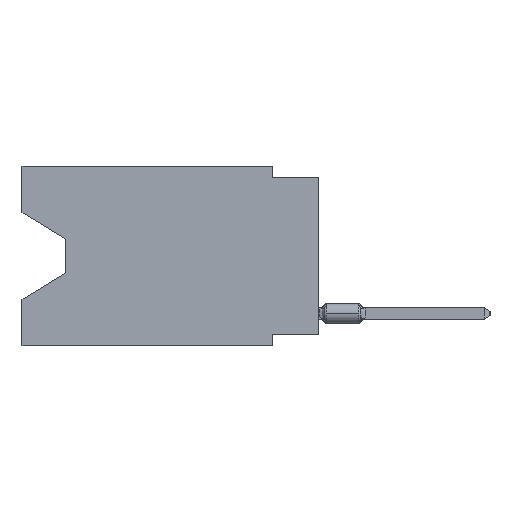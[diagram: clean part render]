
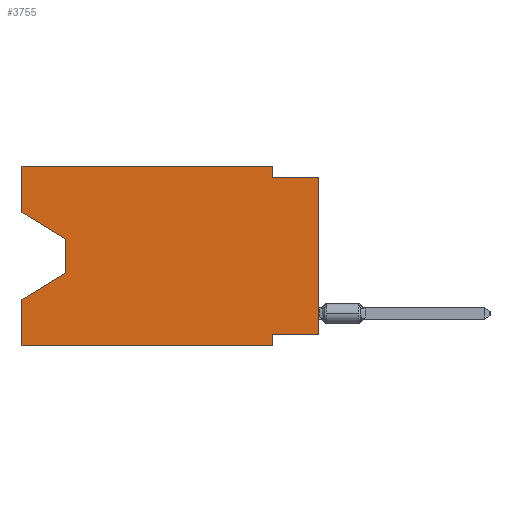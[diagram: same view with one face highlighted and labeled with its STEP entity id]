
A CAD part, left-side view. The second image highlights one B-rep face of the part: STEP entity #3755.
In plain terms, the highlighted planar face has unit normal (-1, 0, 0).
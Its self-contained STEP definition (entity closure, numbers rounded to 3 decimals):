
#475 = CARTESIAN_POINT ( 'NONE',  ( 0., 2.54, -9.906 ) ) ;
#576 = EDGE_CURVE ( 'NONE', #1018, #10502, #11870, .T. ) ;
#692 = ORIENTED_EDGE ( 'NONE', *, *, #12972, .T. ) ;
#781 = EDGE_CURVE ( 'NONE', #21900, #9035, #8437, .T. ) ;
#1018 = VERTEX_POINT ( 'NONE', #19758 ) ;
#1227 = DIRECTION ( 'NONE',  ( 1., 0., 0. ) ) ;
#1311 = LINE ( 'NONE', #3741, #22983 ) ;
#1366 = LINE ( 'NONE', #25809, #26081 ) ;
#2174 = ORIENTED_EDGE ( 'NONE', *, *, #20795, .F. ) ;
#2317 = VERTEX_POINT ( 'NONE', #19214 ) ;
#3523 = DIRECTION ( 'NONE',  ( 0., 0.855, -0.519 ) ) ;
#3629 = LINE ( 'NONE', #17887, #20017 ) ;
#3741 = CARTESIAN_POINT ( 'NONE',  ( 0., 16.383, -9.906 ) ) ;
#3755 = ADVANCED_FACE ( 'NONE', ( #15972 ), #15324, .F. ) ;
#3882 = VECTOR ( 'NONE', #12177, 1000. ) ;
#4515 = EDGE_CURVE ( 'NONE', #24877, #6491, #29339, .T. ) ;
#5330 = LINE ( 'NONE', #24775, #22508 ) ;
#5624 = CARTESIAN_POINT ( 'NONE',  ( 0., 13.97, -5.893 ) ) ;
#6162 = DIRECTION ( 'NONE',  ( 0., 0., -1. ) ) ;
#6491 = VERTEX_POINT ( 'NONE', #12184 ) ;
#6551 = VECTOR ( 'NONE', #9279, 1000. ) ;
#7434 = DIRECTION ( 'NONE',  ( 0., 0., -1. ) ) ;
#7887 = EDGE_CURVE ( 'NONE', #12983, #31976, #1311, .T. ) ;
#8037 = VECTOR ( 'NONE', #14557, 1000. ) ;
#8437 = LINE ( 'NONE', #10877, #13774 ) ;
#9035 = VERTEX_POINT ( 'NONE', #13782 ) ;
#9279 = DIRECTION ( 'NONE',  ( 0., 1., 0. ) ) ;
#9774 = EDGE_LOOP ( 'NONE', ( #692, #27074, #11202, #24869, #21378, #28714, #13624, #13614, #2174, #17462, #12701, #31090 ) ) ;
#9976 = VERTEX_POINT ( 'NONE', #17075 ) ;
#9989 = LINE ( 'NONE', #22144, #13260 ) ;
#10378 = VECTOR ( 'NONE', #13306, 1000. ) ;
#10423 = DIRECTION ( 'NONE',  ( 0., -0.855, -0.519 ) ) ;
#10435 = CARTESIAN_POINT ( 'NONE',  ( 0., 16.383, -2.546 ) ) ;
#10502 = VERTEX_POINT ( 'NONE', #13295 ) ;
#10621 = DIRECTION ( 'NONE',  ( 0., 0., -1. ) ) ;
#10664 = VECTOR ( 'NONE', #3523, 1000. ) ;
#10877 = CARTESIAN_POINT ( 'NONE',  ( 0., 13.97, -4.013 ) ) ;
#11202 = ORIENTED_EDGE ( 'NONE', *, *, #12556, .T. ) ;
#11345 = CARTESIAN_POINT ( 'NONE',  ( 0., 0., -0.635 ) ) ;
#11764 = EDGE_CURVE ( 'NONE', #10502, #31976, #20875, .T. ) ;
#11870 = LINE ( 'NONE', #19007, #6551 ) ;
#12008 = CARTESIAN_POINT ( 'NONE',  ( 0., 2.54, 0. ) ) ;
#12177 = DIRECTION ( 'NONE',  ( 0., 0., 1. ) ) ;
#12184 = CARTESIAN_POINT ( 'NONE',  ( 0., 16.383, 0. ) ) ;
#12424 = EDGE_CURVE ( 'NONE', #1018, #24943, #9989, .T. ) ;
#12425 = DIRECTION ( 'NONE',  ( 0., 0., 1. ) ) ;
#12556 = EDGE_CURVE ( 'NONE', #9035, #9976, #13536, .T. ) ;
#12701 = ORIENTED_EDGE ( 'NONE', *, *, #18022, .F. ) ;
#12972 = EDGE_CURVE ( 'NONE', #24877, #21900, #3629, .T. ) ;
#12983 = VERTEX_POINT ( 'NONE', #20468 ) ;
#13032 = CARTESIAN_POINT ( 'NONE',  ( 0., 0., -0.635 ) ) ;
#13260 = VECTOR ( 'NONE', #12425, 1000. ) ;
#13295 = CARTESIAN_POINT ( 'NONE',  ( 0., 2.54, -9.271 ) ) ;
#13306 = DIRECTION ( 'NONE',  ( 0., -1., 0. ) ) ;
#13536 = LINE ( 'NONE', #5624, #10664 ) ;
#13614 = ORIENTED_EDGE ( 'NONE', *, *, #12424, .T. ) ;
#13624 = ORIENTED_EDGE ( 'NONE', *, *, #576, .F. ) ;
#13770 = LINE ( 'NONE', #11345, #10378 ) ;
#13774 = VECTOR ( 'NONE', #15907, 1000. ) ;
#13782 = CARTESIAN_POINT ( 'NONE',  ( 0., 13.97, -5.893 ) ) ;
#14557 = DIRECTION ( 'NONE',  ( 0., -1., 0. ) ) ;
#15324 = PLANE ( 'NONE',  #20404 ) ;
#15907 = DIRECTION ( 'NONE',  ( 0., 0., -1. ) ) ;
#15972 = FACE_OUTER_BOUND ( 'NONE', #9774, .T. ) ;
#16361 = CARTESIAN_POINT ( 'NONE',  ( 0., 2.54, -9.906 ) ) ;
#17075 = CARTESIAN_POINT ( 'NONE',  ( 0., 16.383, -7.36 ) ) ;
#17462 = ORIENTED_EDGE ( 'NONE', *, *, #22603, .F. ) ;
#17483 = CARTESIAN_POINT ( 'NONE',  ( 0., 16.383, 0. ) ) ;
#17887 = CARTESIAN_POINT ( 'NONE',  ( 0., 16.383, -2.546 ) ) ;
#17965 = VECTOR ( 'NONE', #6162, 1000. ) ;
#18022 = EDGE_CURVE ( 'NONE', #6491, #31521, #19738, .T. ) ;
#18237 = CARTESIAN_POINT ( 'NONE',  ( 0., 16.383, 0. ) ) ;
#19007 = CARTESIAN_POINT ( 'NONE',  ( 0., 0., -9.271 ) ) ;
#19214 = CARTESIAN_POINT ( 'NONE',  ( 0., 2.54, -0.635 ) ) ;
#19293 = CARTESIAN_POINT ( 'NONE',  ( 0., 16.383, 0. ) ) ;
#19738 = LINE ( 'NONE', #17483, #8037 ) ;
#19758 = CARTESIAN_POINT ( 'NONE',  ( 0., 0., -9.271 ) ) ;
#20017 = VECTOR ( 'NONE', #10423, 1000. ) ;
#20404 = AXIS2_PLACEMENT_3D ( 'NONE', #18237, #1227, #10621 ) ;
#20468 = CARTESIAN_POINT ( 'NONE',  ( 0., 16.383, -9.906 ) ) ;
#20795 = EDGE_CURVE ( 'NONE', #2317, #24943, #13770, .T. ) ;
#20875 = LINE ( 'NONE', #16361, #17965 ) ;
#21378 = ORIENTED_EDGE ( 'NONE', *, *, #7887, .T. ) ;
#21900 = VERTEX_POINT ( 'NONE', #24559 ) ;
#22144 = CARTESIAN_POINT ( 'NONE',  ( 0., 0., 0. ) ) ;
#22508 = VECTOR ( 'NONE', #7434, 1000. ) ;
#22603 = EDGE_CURVE ( 'NONE', #31521, #2317, #5330, .T. ) ;
#22983 = VECTOR ( 'NONE', #30928, 1000. ) ;
#24559 = CARTESIAN_POINT ( 'NONE',  ( 0., 13.97, -4.013 ) ) ;
#24775 = CARTESIAN_POINT ( 'NONE',  ( 0., 2.54, 0. ) ) ;
#24869 = ORIENTED_EDGE ( 'NONE', *, *, #25081, .F. ) ;
#24877 = VERTEX_POINT ( 'NONE', #10435 ) ;
#24943 = VERTEX_POINT ( 'NONE', #13032 ) ;
#25081 = EDGE_CURVE ( 'NONE', #12983, #9976, #1366, .T. ) ;
#25809 = CARTESIAN_POINT ( 'NONE',  ( 0., 16.383, 0. ) ) ;
#26081 = VECTOR ( 'NONE', #28868, 1000. ) ;
#27074 = ORIENTED_EDGE ( 'NONE', *, *, #781, .T. ) ;
#28714 = ORIENTED_EDGE ( 'NONE', *, *, #11764, .F. ) ;
#28868 = DIRECTION ( 'NONE',  ( 0., 0., 1. ) ) ;
#29339 = LINE ( 'NONE', #19293, #3882 ) ;
#30928 = DIRECTION ( 'NONE',  ( 0., -1., 0. ) ) ;
#31090 = ORIENTED_EDGE ( 'NONE', *, *, #4515, .F. ) ;
#31521 = VERTEX_POINT ( 'NONE', #12008 ) ;
#31976 = VERTEX_POINT ( 'NONE', #475 ) ;
